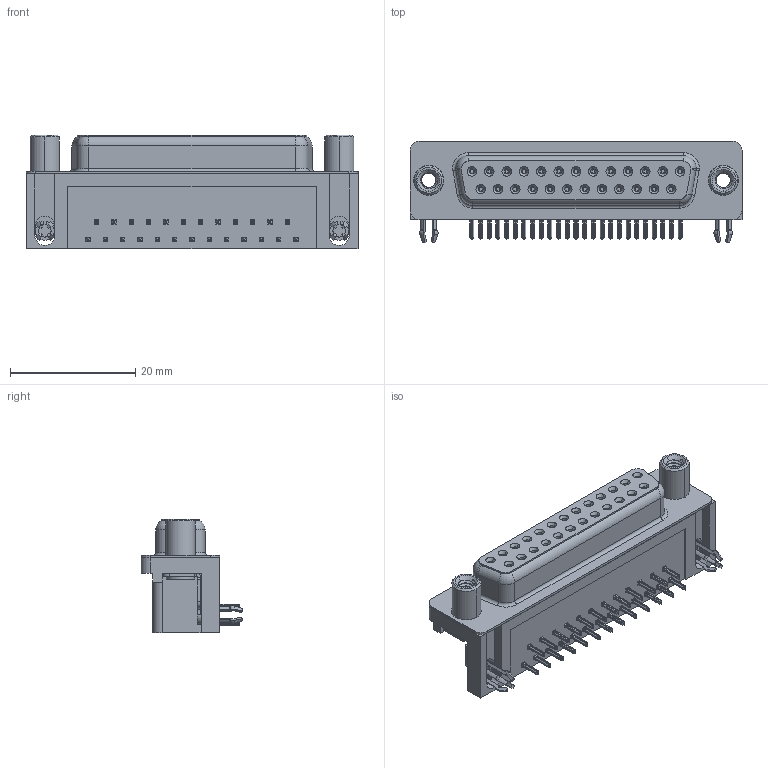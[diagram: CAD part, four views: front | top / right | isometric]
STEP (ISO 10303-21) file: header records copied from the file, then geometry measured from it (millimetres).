
FILE_DESCRIPTION (( 'STEP AP203' ), '1' );
FILE_NAME ('622-025-668-040.STEP', '2019-11-20T05:14:55', ( '' ), ( '' ), 'SwSTEP 2.0', 'SolidWorks 2016', '' );
FILE_SCHEMA (( 'CONFIG_CONTROL_DESIGN' ));
Length unit declared in the file: millimetre
Products named in the file (7): 622-025-668-040; 622 4 Prong Board Lock; 622 Socket Bottom; 622 Contact Top; 622 Housing_25 Socket; 622 Shell_25 Socket; 622 Round Threaded Standoff
Assembly tree (31 placements, depth 2):
  622-025-668-040
    622 Housing_25 Socket
    622 Shell_25 Socket
    622 Socket Bottom  x12
    622 Contact Top  x13
    622 4 Prong Board Lock  x2
    622 Round Threaded Standoff  x2
Bounding box: 53.04 x 16.25 x 18.2 mm (x, y, z)
Volume: 7702.8 mm3; surface area: 9714.6 mm2
Topology: 31 solids, 31 shells, 3966 faces, 10466 edges, 6580 vertices
Faces by surface type: plane 1758, cylinder 934, bspline 868, cone 352, torus 54
Entity records: 33133 total; most frequent: CARTESIAN_POINT 10265, ORIENTED_EDGE 4572, DIRECTION 4219, EDGE_CURVE 2286, VERTEX_POINT 1466, LINE 1449, VECTOR 1449, AXIS2_PLACEMENT_3D 1385
